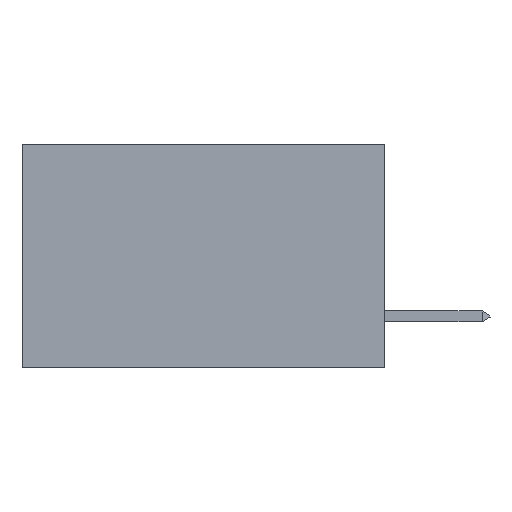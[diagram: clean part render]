
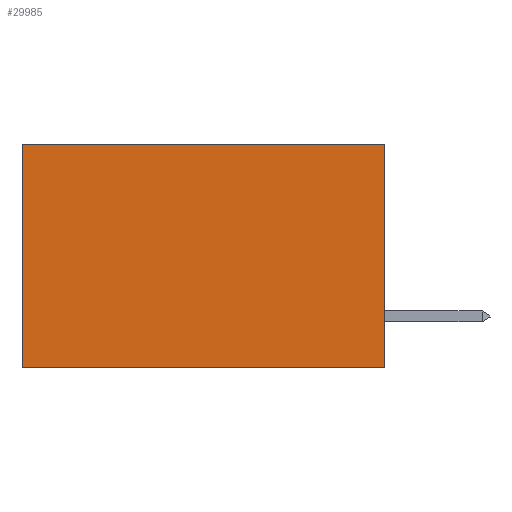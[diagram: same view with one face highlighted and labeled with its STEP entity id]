
A CAD part, left-side view. The second image highlights one B-rep face of the part: STEP entity #29985.
In plain terms, the highlighted planar face has unit normal (-1, 0, 0).
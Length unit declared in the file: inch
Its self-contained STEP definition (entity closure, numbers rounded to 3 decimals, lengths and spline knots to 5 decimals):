
#1015 = DIRECTION ( 'NONE',  ( 0., 1., 0. ) ) ;
#1738 = VERTEX_POINT ( 'NONE', #21719 ) ;
#2136 = VECTOR ( 'NONE', #33004, 39.37008 ) ;
#2431 = ORIENTED_EDGE ( 'NONE', *, *, #31696, .T. ) ;
#3654 = CARTESIAN_POINT ( 'NONE',  ( 0.2875, 0., -0.37 ) ) ;
#3896 = VECTOR ( 'NONE', #1015, 39.37008 ) ;
#4659 = ORIENTED_EDGE ( 'NONE', *, *, #24118, .F. ) ;
#4670 = DIRECTION ( 'NONE',  ( 0., 1., 0. ) ) ;
#6582 = CARTESIAN_POINT ( 'NONE',  ( 0.2875, 0., -0.37 ) ) ;
#11538 = LINE ( 'NONE', #3654, #3896 ) ;
#11722 = FACE_OUTER_BOUND ( 'NONE', #34237, .T. ) ;
#12888 = CARTESIAN_POINT ( 'NONE',  ( 0.2875, 0., 0. ) ) ;
#14451 = DIRECTION ( 'NONE',  ( 0., 0., -1. ) ) ;
#14980 = EDGE_CURVE ( 'NONE', #16805, #18140, #32943, .T. ) ;
#15656 = LINE ( 'NONE', #24380, #29899 ) ;
#16805 = VERTEX_POINT ( 'NONE', #25704 ) ;
#17018 = VECTOR ( 'NONE', #14451, 39.37008 ) ;
#17314 = DIRECTION ( 'NONE',  ( 1., 0., 0. ) ) ;
#17525 = CARTESIAN_POINT ( 'NONE',  ( 0.2875, 0., 0. ) ) ;
#18140 = VERTEX_POINT ( 'NONE', #6582 ) ;
#21719 = CARTESIAN_POINT ( 'NONE',  ( 0.2875, 0.6, -0.37 ) ) ;
#24118 = EDGE_CURVE ( 'NONE', #18140, #1738, #11538, .T. ) ;
#24380 = CARTESIAN_POINT ( 'NONE',  ( 0.2875, 0., 0. ) ) ;
#25106 = VERTEX_POINT ( 'NONE', #28514 ) ;
#25704 = CARTESIAN_POINT ( 'NONE',  ( 0.2875, 0., 0. ) ) ;
#27677 = ORIENTED_EDGE ( 'NONE', *, *, #14980, .F. ) ;
#28514 = CARTESIAN_POINT ( 'NONE',  ( 0.2875, 0.6, 0. ) ) ;
#28929 = LINE ( 'NONE', #31555, #17018 ) ;
#29899 = VECTOR ( 'NONE', #4670, 39.37008 ) ;
#29985 = ADVANCED_FACE ( 'NONE', ( #11722 ), #31530, .F. ) ;
#30759 = ORIENTED_EDGE ( 'NONE', *, *, #31946, .T. ) ;
#31530 = PLANE ( 'NONE',  #35990 ) ;
#31555 = CARTESIAN_POINT ( 'NONE',  ( 0.2875, 0.6, 0. ) ) ;
#31696 = EDGE_CURVE ( 'NONE', #16805, #25106, #15656, .T. ) ;
#31946 = EDGE_CURVE ( 'NONE', #25106, #1738, #28929, .T. ) ;
#32116 = DIRECTION ( 'NONE',  ( 0., 0., -1. ) ) ;
#32943 = LINE ( 'NONE', #12888, #2136 ) ;
#33004 = DIRECTION ( 'NONE',  ( 0., 0., -1. ) ) ;
#34237 = EDGE_LOOP ( 'NONE', ( #30759, #4659, #27677, #2431 ) ) ;
#35990 = AXIS2_PLACEMENT_3D ( 'NONE', #17525, #17314, #32116 ) ;
